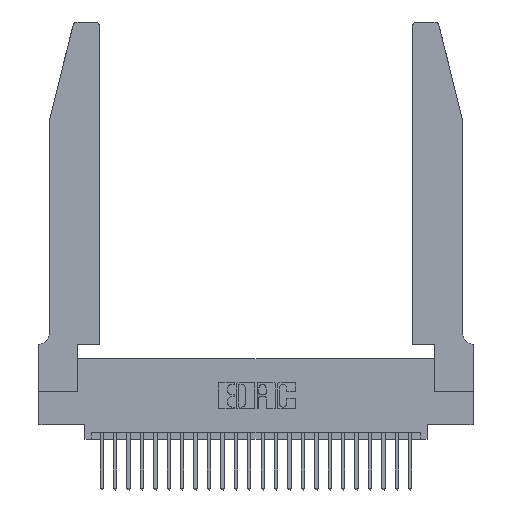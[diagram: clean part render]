
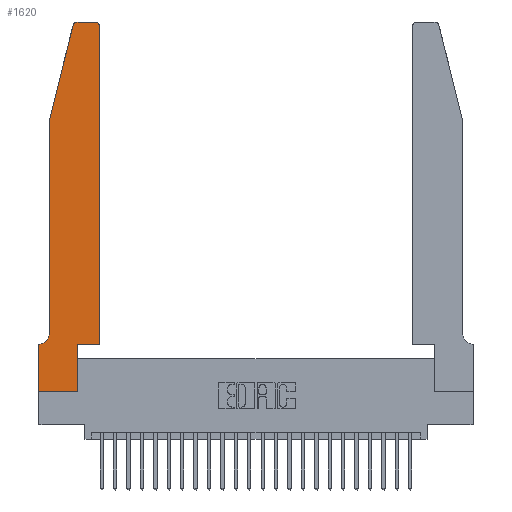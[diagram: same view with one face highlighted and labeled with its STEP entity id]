
A CAD part, top view. The second image highlights one B-rep face of the part: STEP entity #1620.
In plain terms, the highlighted planar face has unit normal (0, 0, 1).
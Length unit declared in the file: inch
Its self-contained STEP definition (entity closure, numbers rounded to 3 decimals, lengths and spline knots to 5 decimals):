
#174 = CARTESIAN_POINT ( 'NONE',  ( 0.4505, 0.35, 0.37 ) ) ;
#643 = ORIENTED_EDGE ( 'NONE', *, *, #5323, .T. ) ;
#894 = EDGE_CURVE ( 'NONE', #12690, #12081, #20989, .T. ) ;
#948 = CARTESIAN_POINT ( 'NONE',  ( 0.0755, 2., 0.37 ) ) ;
#970 = VERTEX_POINT ( 'NONE', #11969 ) ;
#1039 = ORIENTED_EDGE ( 'NONE', *, *, #11760, .T. ) ;
#1088 = LINE ( 'NONE', #174, #9364 ) ;
#1460 = CARTESIAN_POINT ( 'NONE',  ( 0.0755, 0.42, 0.37 ) ) ;
#1620 = ADVANCED_FACE ( 'NONE', ( #7411 ), #7613, .T. ) ;
#1786 = DIRECTION ( 'NONE',  ( 0., -1., 0. ) ) ;
#2214 = ORIENTED_EDGE ( 'NONE', *, *, #20144, .T. ) ;
#2231 = CARTESIAN_POINT ( 'NONE',  ( 0., 0., 0.37 ) ) ;
#3152 = DIRECTION ( 'NONE',  ( -1., 0., 0. ) ) ;
#3202 = DIRECTION ( 'NONE',  ( -1., 0., 0. ) ) ;
#3583 = DIRECTION ( 'NONE',  ( 0., -1., 0. ) ) ;
#4162 = CARTESIAN_POINT ( 'NONE',  ( 0.4205, 2.75, 0.37 ) ) ;
#4859 = VERTEX_POINT ( 'NONE', #1460 ) ;
#4875 = CARTESIAN_POINT ( 'NONE',  ( 0.0755, 0.35, 0.37 ) ) ;
#5164 = CARTESIAN_POINT ( 'NONE',  ( 0.2605, 2.75, 0.37 ) ) ;
#5323 = EDGE_CURVE ( 'NONE', #23924, #19878, #25842, .T. ) ;
#5508 = CARTESIAN_POINT ( 'NONE',  ( 0.284, 2.75, 0.37 ) ) ;
#5536 = LINE ( 'NONE', #7859, #6443 ) ;
#5609 = AXIS2_PLACEMENT_3D ( 'NONE', #7259, #25508, #3152 ) ;
#5619 = VERTEX_POINT ( 'NONE', #6327 ) ;
#5828 = LINE ( 'NONE', #10875, #6792 ) ;
#5980 = ORIENTED_EDGE ( 'NONE', *, *, #894, .T. ) ;
#6174 = LINE ( 'NONE', #2231, #21704 ) ;
#6327 = CARTESIAN_POINT ( 'NONE',  ( 0.0055, 0.35, 0.37 ) ) ;
#6350 = ORIENTED_EDGE ( 'NONE', *, *, #18407, .T. ) ;
#6389 = CIRCLE ( 'NONE', #8748, 0.03 ) ;
#6443 = VECTOR ( 'NONE', #1786, 39.37008 ) ;
#6706 = EDGE_CURVE ( 'NONE', #19878, #16548, #1088, .T. ) ;
#6792 = VECTOR ( 'NONE', #10966, 39.37008 ) ;
#7228 = VECTOR ( 'NONE', #25337, 39.37008 ) ;
#7259 = CARTESIAN_POINT ( 'NONE',  ( 0.0055, 0.42, 0.37 ) ) ;
#7411 = FACE_OUTER_BOUND ( 'NONE', #22026, .T. ) ;
#7613 = PLANE ( 'NONE',  #10660 ) ;
#7859 = CARTESIAN_POINT ( 'NONE',  ( 0., 0., 0.37 ) ) ;
#8437 = ORIENTED_EDGE ( 'NONE', *, *, #6706, .T. ) ;
#8605 = VECTOR ( 'NONE', #15541, 39.37008 ) ;
#8748 = AXIS2_PLACEMENT_3D ( 'NONE', #25105, #13060, #17198 ) ;
#9291 = ORIENTED_EDGE ( 'NONE', *, *, #12336, .T. ) ;
#9364 = VECTOR ( 'NONE', #16954, 39.37008 ) ;
#10660 = AXIS2_PLACEMENT_3D ( 'NONE', #15418, #23512, #17520 ) ;
#10875 = CARTESIAN_POINT ( 'NONE',  ( 0.2865, 0.35, 0.37 ) ) ;
#10966 = DIRECTION ( 'NONE',  ( 0., 1., 0. ) ) ;
#11676 = CARTESIAN_POINT ( 'NONE',  ( 0.4205, 2.72, 0.37 ) ) ;
#11760 = EDGE_CURVE ( 'NONE', #24132, #4859, #19416, .T. ) ;
#11948 = CARTESIAN_POINT ( 'NONE',  ( 0.0755, 2., 0.37 ) ) ;
#11969 = CARTESIAN_POINT ( 'NONE',  ( 0.2865, 0., 0.37 ) ) ;
#12081 = VERTEX_POINT ( 'NONE', #5508 ) ;
#12336 = EDGE_CURVE ( 'NONE', #12081, #21148, #6389, .T. ) ;
#12479 = VECTOR ( 'NONE', #3583, 39.37008 ) ;
#12690 = VERTEX_POINT ( 'NONE', #4162 ) ;
#12919 = EDGE_CURVE ( 'NONE', #5619, #16765, #19355, .T. ) ;
#13060 = DIRECTION ( 'NONE',  ( 0., 0., 1. ) ) ;
#13331 = LINE ( 'NONE', #948, #18340 ) ;
#13466 = DIRECTION ( 'NONE',  ( 1., 0., 0. ) ) ;
#13516 = ORIENTED_EDGE ( 'NONE', *, *, #22218, .T. ) ;
#14200 = CIRCLE ( 'NONE', #5609, 0.07 ) ;
#15418 = CARTESIAN_POINT ( 'NONE',  ( 0., 0.35, 0.37 ) ) ;
#15465 = ORIENTED_EDGE ( 'NONE', *, *, #17572, .T. ) ;
#15541 = DIRECTION ( 'NONE',  ( -1., 0., 0. ) ) ;
#15675 = DIRECTION ( 'NONE',  ( 0., 0., 1. ) ) ;
#16145 = CARTESIAN_POINT ( 'NONE',  ( 0.25487, 2.72718, 0.37 ) ) ;
#16319 = ORIENTED_EDGE ( 'NONE', *, *, #22394, .T. ) ;
#16548 = VERTEX_POINT ( 'NONE', #22770 ) ;
#16765 = VERTEX_POINT ( 'NONE', #19424 ) ;
#16898 = VECTOR ( 'NONE', #3202, 39.37008 ) ;
#16954 = DIRECTION ( 'NONE',  ( 0., 1., 0. ) ) ;
#17150 = CARTESIAN_POINT ( 'NONE',  ( 0.4505, 0.35, 0.37 ) ) ;
#17198 = DIRECTION ( 'NONE',  ( 1., 0., 0. ) ) ;
#17274 = CARTESIAN_POINT ( 'NONE',  ( 0.2865, 0.35, 0.37 ) ) ;
#17520 = DIRECTION ( 'NONE',  ( 1., 0., 0. ) ) ;
#17572 = EDGE_CURVE ( 'NONE', #21148, #24132, #13331, .T. ) ;
#18209 = AXIS2_PLACEMENT_3D ( 'NONE', #11676, #15675, #13466 ) ;
#18340 = VECTOR ( 'NONE', #22995, 39.37008 ) ;
#18407 = EDGE_CURVE ( 'NONE', #4859, #5619, #14200, .T. ) ;
#19116 = CIRCLE ( 'NONE', #18209, 0.03 ) ;
#19211 = CARTESIAN_POINT ( 'NONE',  ( 0., 0., 0.37 ) ) ;
#19291 = ORIENTED_EDGE ( 'NONE', *, *, #12919, .T. ) ;
#19355 = LINE ( 'NONE', #4875, #8605 ) ;
#19416 = LINE ( 'NONE', #20118, #12479 ) ;
#19424 = CARTESIAN_POINT ( 'NONE',  ( 0., 0.35, 0.37 ) ) ;
#19878 = VERTEX_POINT ( 'NONE', #23145 ) ;
#20118 = CARTESIAN_POINT ( 'NONE',  ( 0.0755, 2., 0.37 ) ) ;
#20144 = EDGE_CURVE ( 'NONE', #22935, #970, #6174, .T. ) ;
#20583 = DIRECTION ( 'NONE',  ( 1., 0., 0. ) ) ;
#20989 = LINE ( 'NONE', #5164, #16898 ) ;
#21148 = VERTEX_POINT ( 'NONE', #16145 ) ;
#21704 = VECTOR ( 'NONE', #20583, 39.37008 ) ;
#22026 = EDGE_LOOP ( 'NONE', ( #5980, #9291, #15465, #1039, #6350, #19291, #16319, #2214, #13516, #643, #8437, #24972 ) ) ;
#22218 = EDGE_CURVE ( 'NONE', #970, #23924, #5828, .T. ) ;
#22226 = EDGE_CURVE ( 'NONE', #16548, #12690, #19116, .T. ) ;
#22394 = EDGE_CURVE ( 'NONE', #16765, #22935, #5536, .T. ) ;
#22770 = CARTESIAN_POINT ( 'NONE',  ( 0.4505, 2.72, 0.37 ) ) ;
#22935 = VERTEX_POINT ( 'NONE', #19211 ) ;
#22995 = DIRECTION ( 'NONE',  ( -0.239, -0.971, 0. ) ) ;
#23145 = CARTESIAN_POINT ( 'NONE',  ( 0.4505, 0.35, 0.37 ) ) ;
#23512 = DIRECTION ( 'NONE',  ( 0., 0., 1. ) ) ;
#23924 = VERTEX_POINT ( 'NONE', #17274 ) ;
#24132 = VERTEX_POINT ( 'NONE', #11948 ) ;
#24972 = ORIENTED_EDGE ( 'NONE', *, *, #22226, .T. ) ;
#25105 = CARTESIAN_POINT ( 'NONE',  ( 0.284, 2.72, 0.37 ) ) ;
#25337 = DIRECTION ( 'NONE',  ( 1., 0., 0. ) ) ;
#25508 = DIRECTION ( 'NONE',  ( 0., 0., -1. ) ) ;
#25842 = LINE ( 'NONE', #17150, #7228 ) ;
